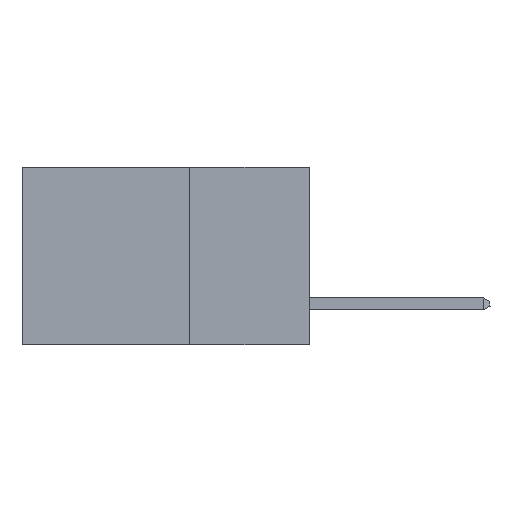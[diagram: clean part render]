
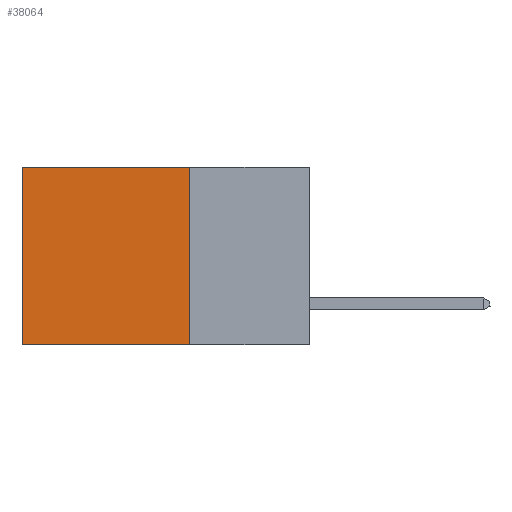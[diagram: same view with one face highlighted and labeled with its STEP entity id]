
A CAD part, left-side view. The second image highlights one B-rep face of the part: STEP entity #38064.
In plain terms, the highlighted planar face has unit normal (-1, 0, 0).
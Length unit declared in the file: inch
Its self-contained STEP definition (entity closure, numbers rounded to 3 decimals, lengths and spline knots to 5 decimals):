
#220 = LINE ( 'NONE', #35371, #33340 ) ;
#762 = DIRECTION ( 'NONE',  ( 0., 1., 0. ) ) ;
#3596 = LINE ( 'NONE', #16905, #19630 ) ;
#3674 = LINE ( 'NONE', #23253, #17725 ) ;
#3710 = CARTESIAN_POINT ( 'NONE',  ( 0.2875, 0.6, -0.37 ) ) ;
#3990 = VERTEX_POINT ( 'NONE', #31577 ) ;
#5375 = LINE ( 'NONE', #24878, #16766 ) ;
#5668 = ORIENTED_EDGE ( 'NONE', *, *, #38305, .F. ) ;
#6068 = VERTEX_POINT ( 'NONE', #8673 ) ;
#7332 = DIRECTION ( 'NONE',  ( 0., 0., -1. ) ) ;
#8673 = CARTESIAN_POINT ( 'NONE',  ( 0.2875, 0.25, 0. ) ) ;
#9253 = VERTEX_POINT ( 'NONE', #3710 ) ;
#10108 = VERTEX_POINT ( 'NONE', #30175 ) ;
#12859 = EDGE_CURVE ( 'NONE', #3990, #9253, #5375, .T. ) ;
#14012 = ORIENTED_EDGE ( 'NONE', *, *, #12859, .T. ) ;
#14464 = FACE_OUTER_BOUND ( 'NONE', #19116, .T. ) ;
#15576 = PLANE ( 'NONE',  #19649 ) ;
#16766 = VECTOR ( 'NONE', #25157, 39.37008 ) ;
#16905 = CARTESIAN_POINT ( 'NONE',  ( 0.2875, 0.25, -0.37 ) ) ;
#17725 = VECTOR ( 'NONE', #7332, 39.37008 ) ;
#18533 = DIRECTION ( 'NONE',  ( 1., 0., 0. ) ) ;
#18815 = CARTESIAN_POINT ( 'NONE',  ( 0.2875, 0.25, 0. ) ) ;
#18878 = EDGE_CURVE ( 'NONE', #6068, #3990, #220, .T. ) ;
#19116 = EDGE_LOOP ( 'NONE', ( #14012, #5668, #19510, #37062 ) ) ;
#19510 = ORIENTED_EDGE ( 'NONE', *, *, #24323, .F. ) ;
#19630 = VECTOR ( 'NONE', #762, 39.37008 ) ;
#19649 = AXIS2_PLACEMENT_3D ( 'NONE', #18815, #18533, #34623 ) ;
#23253 = CARTESIAN_POINT ( 'NONE',  ( 0.2875, 0.25, 0. ) ) ;
#24323 = EDGE_CURVE ( 'NONE', #6068, #10108, #3674, .T. ) ;
#24878 = CARTESIAN_POINT ( 'NONE',  ( 0.2875, 0.6, 0. ) ) ;
#25157 = DIRECTION ( 'NONE',  ( 0., 0., -1. ) ) ;
#25650 = DIRECTION ( 'NONE',  ( 0., 1., 0. ) ) ;
#30175 = CARTESIAN_POINT ( 'NONE',  ( 0.2875, 0.25, -0.37 ) ) ;
#31577 = CARTESIAN_POINT ( 'NONE',  ( 0.2875, 0.6, 0. ) ) ;
#33340 = VECTOR ( 'NONE', #25650, 39.37008 ) ;
#34623 = DIRECTION ( 'NONE',  ( 0., 0., -1. ) ) ;
#35371 = CARTESIAN_POINT ( 'NONE',  ( 0.2875, 0.25, 0. ) ) ;
#37062 = ORIENTED_EDGE ( 'NONE', *, *, #18878, .T. ) ;
#38064 = ADVANCED_FACE ( 'NONE', ( #14464 ), #15576, .F. ) ;
#38305 = EDGE_CURVE ( 'NONE', #10108, #9253, #3596, .T. ) ;
